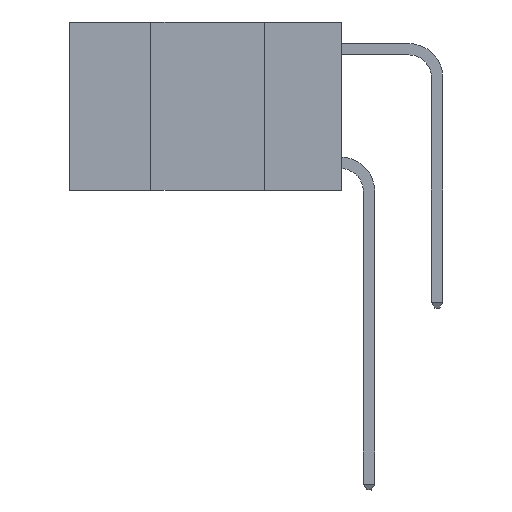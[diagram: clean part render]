
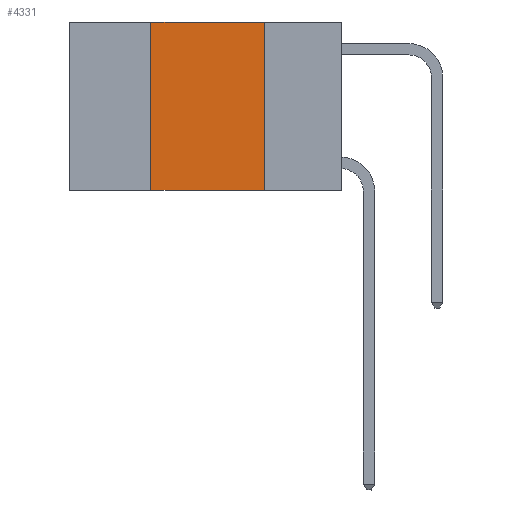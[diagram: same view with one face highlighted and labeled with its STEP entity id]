
A CAD part, left-side view. The second image highlights one B-rep face of the part: STEP entity #4331.
In plain terms, the highlighted planar face has unit normal (-1, 0, 0).
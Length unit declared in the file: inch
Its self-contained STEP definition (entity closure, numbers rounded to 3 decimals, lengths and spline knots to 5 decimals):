
#822 = LINE ( 'NONE', #17229, #17125 ) ;
#1010 = DIRECTION ( 'NONE',  ( 1., 0., 0. ) ) ;
#1046 = EDGE_CURVE ( 'NONE', #16080, #4900, #2692, .T. ) ;
#1446 = CARTESIAN_POINT ( 'NONE',  ( 0., 0.42, 0. ) ) ;
#2540 = ORIENTED_EDGE ( 'NONE', *, *, #1046, .F. ) ;
#2692 = LINE ( 'NONE', #11749, #9819 ) ;
#4090 = LINE ( 'NONE', #19033, #12245 ) ;
#4331 = ADVANCED_FACE ( 'NONE', ( #18862 ), #20513, .F. ) ;
#4874 = CARTESIAN_POINT ( 'NONE',  ( 0., 0.17, -0.37 ) ) ;
#4900 = VERTEX_POINT ( 'NONE', #7197 ) ;
#5876 = ORIENTED_EDGE ( 'NONE', *, *, #6740, .F. ) ;
#6073 = DIRECTION ( 'NONE',  ( 0., 0., -1. ) ) ;
#6535 = LINE ( 'NONE', #18238, #9355 ) ;
#6740 = EDGE_CURVE ( 'NONE', #4900, #18757, #4090, .T. ) ;
#6901 = DIRECTION ( 'NONE',  ( 0., -1., 0. ) ) ;
#7197 = CARTESIAN_POINT ( 'NONE',  ( 0., 0.17, 0. ) ) ;
#8940 = EDGE_CURVE ( 'NONE', #12427, #16080, #6535, .T. ) ;
#9355 = VECTOR ( 'NONE', #10042, 39.37008 ) ;
#9819 = VECTOR ( 'NONE', #6901, 39.37008 ) ;
#10042 = DIRECTION ( 'NONE',  ( 0., 0., 1. ) ) ;
#11124 = EDGE_CURVE ( 'NONE', #12427, #18757, #822, .T. ) ;
#11217 = AXIS2_PLACEMENT_3D ( 'NONE', #18838, #1010, #12445 ) ;
#11218 = ORIENTED_EDGE ( 'NONE', *, *, #8940, .F. ) ;
#11749 = CARTESIAN_POINT ( 'NONE',  ( 0., 0.6, 0. ) ) ;
#12245 = VECTOR ( 'NONE', #6073, 39.37008 ) ;
#12427 = VERTEX_POINT ( 'NONE', #17735 ) ;
#12445 = DIRECTION ( 'NONE',  ( 0., 0., -1. ) ) ;
#16080 = VERTEX_POINT ( 'NONE', #1446 ) ;
#17125 = VECTOR ( 'NONE', #18893, 39.37008 ) ;
#17229 = CARTESIAN_POINT ( 'NONE',  ( 0., 0.6, -0.37 ) ) ;
#17735 = CARTESIAN_POINT ( 'NONE',  ( 0., 0.42, -0.37 ) ) ;
#18238 = CARTESIAN_POINT ( 'NONE',  ( 0., 0.42, 0. ) ) ;
#18757 = VERTEX_POINT ( 'NONE', #4874 ) ;
#18838 = CARTESIAN_POINT ( 'NONE',  ( 0., 0.6, 0. ) ) ;
#18862 = FACE_OUTER_BOUND ( 'NONE', #19018, .T. ) ;
#18893 = DIRECTION ( 'NONE',  ( 0., -1., 0. ) ) ;
#19018 = EDGE_LOOP ( 'NONE', ( #5876, #2540, #11218, #19851 ) ) ;
#19033 = CARTESIAN_POINT ( 'NONE',  ( 0., 0.17, 0. ) ) ;
#19851 = ORIENTED_EDGE ( 'NONE', *, *, #11124, .T. ) ;
#20513 = PLANE ( 'NONE',  #11217 ) ;
